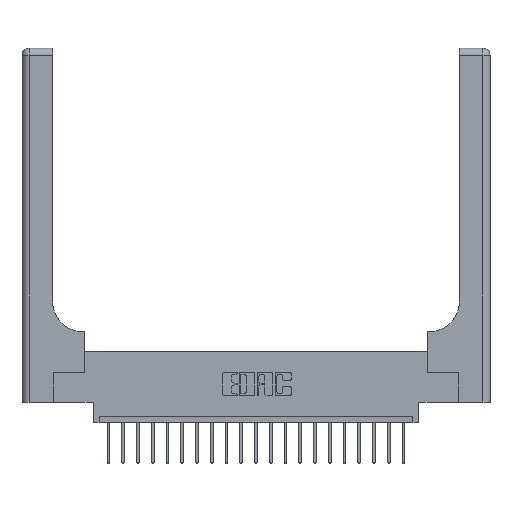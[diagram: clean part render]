
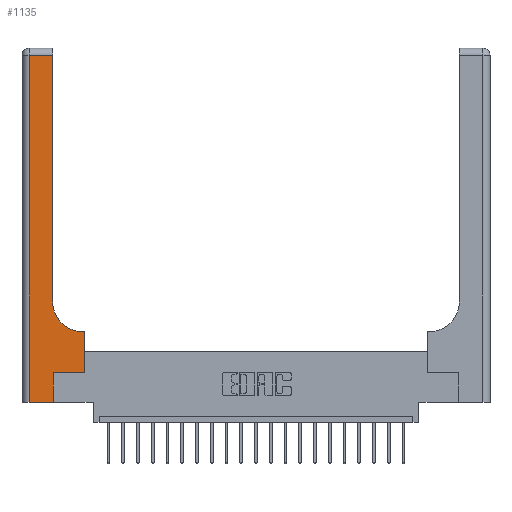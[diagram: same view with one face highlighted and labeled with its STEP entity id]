
A CAD part, top view. The second image highlights one B-rep face of the part: STEP entity #1135.
In plain terms, the highlighted planar face has unit normal (0, 0, 1).
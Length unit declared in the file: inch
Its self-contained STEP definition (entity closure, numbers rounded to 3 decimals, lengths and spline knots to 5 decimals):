
#511 = FACE_OUTER_BOUND ( 'NONE', #14439, .T. ) ;
#1135 = ADVANCED_FACE ( 'NONE', ( #511 ), #15843, .F. ) ;
#1681 = LINE ( 'NONE', #21353, #6158 ) ;
#1889 = CIRCLE ( 'NONE', #6447, 0.25 ) ;
#1968 = VECTOR ( 'NONE', #11763, 39.37008 ) ;
#2042 = CARTESIAN_POINT ( 'NONE',  ( 0.265, 0., 0.37 ) ) ;
#2161 = EDGE_CURVE ( 'NONE', #17078, #8652, #13279, .T. ) ;
#2388 = LINE ( 'NONE', #4135, #10143 ) ;
#3120 = ORIENTED_EDGE ( 'NONE', *, *, #17244, .T. ) ;
#3235 = VERTEX_POINT ( 'NONE', #18575 ) ;
#3741 = LINE ( 'NONE', #19071, #19484 ) ;
#4117 = CARTESIAN_POINT ( 'NONE',  ( 0.26, 2.94, 0.37 ) ) ;
#4135 = CARTESIAN_POINT ( 'NONE',  ( 0.265, 0.25, 0.37 ) ) ;
#4670 = VECTOR ( 'NONE', #9063, 39.37008 ) ;
#5354 = VERTEX_POINT ( 'NONE', #17963 ) ;
#5547 = EDGE_CURVE ( 'NONE', #6151, #3235, #2388, .T. ) ;
#5849 = VERTEX_POINT ( 'NONE', #21600 ) ;
#6035 = CARTESIAN_POINT ( 'NONE',  ( 0.26, 0.85, 0.37 ) ) ;
#6151 = VERTEX_POINT ( 'NONE', #16131 ) ;
#6158 = VECTOR ( 'NONE', #18116, 39.37008 ) ;
#6335 = AXIS2_PLACEMENT_3D ( 'NONE', #19245, #17715, #14543 ) ;
#6447 = AXIS2_PLACEMENT_3D ( 'NONE', #14978, #6541, #6746 ) ;
#6541 = DIRECTION ( 'NONE',  ( 0., 0., -1. ) ) ;
#6746 = DIRECTION ( 'NONE',  ( 1., 0., 0. ) ) ;
#8096 = EDGE_CURVE ( 'NONE', #8652, #5354, #3741, .T. ) ;
#8153 = ORIENTED_EDGE ( 'NONE', *, *, #15466, .T. ) ;
#8238 = CARTESIAN_POINT ( 'NONE',  ( 0., 2.94, 0.37 ) ) ;
#8451 = CARTESIAN_POINT ( 'NONE',  ( 0.265, 0., 0.37 ) ) ;
#8599 = VECTOR ( 'NONE', #13018, 39.37008 ) ;
#8652 = VERTEX_POINT ( 'NONE', #20749 ) ;
#8742 = LINE ( 'NONE', #17387, #4670 ) ;
#9063 = DIRECTION ( 'NONE',  ( 0., 1., 0. ) ) ;
#10143 = VECTOR ( 'NONE', #20635, 39.37008 ) ;
#10161 = EDGE_CURVE ( 'NONE', #17008, #6151, #20239, .T. ) ;
#10451 = DIRECTION ( 'NONE',  ( 0., 1., 0. ) ) ;
#11394 = CARTESIAN_POINT ( 'NONE',  ( 0.26, 0.6, 0.37 ) ) ;
#11500 = VERTEX_POINT ( 'NONE', #6035 ) ;
#11763 = DIRECTION ( 'NONE',  ( 0., 1., 0. ) ) ;
#13018 = DIRECTION ( 'NONE',  ( -1., 0., 0. ) ) ;
#13279 = LINE ( 'NONE', #8238, #16846 ) ;
#13583 = ORIENTED_EDGE ( 'NONE', *, *, #8096, .T. ) ;
#14439 = EDGE_LOOP ( 'NONE', ( #15401, #19778, #13583, #3120, #19257, #15819, #18914, #16451, #8153 ) ) ;
#14543 = DIRECTION ( 'NONE',  ( -1., 0., 0. ) ) ;
#14787 = CARTESIAN_POINT ( 'NONE',  ( 0.51, 0.6, 0.37 ) ) ;
#14978 = CARTESIAN_POINT ( 'NONE',  ( 0.51, 0.85, 0.37 ) ) ;
#15192 = EDGE_CURVE ( 'NONE', #3235, #5849, #8742, .T. ) ;
#15267 = LINE ( 'NONE', #11394, #8599 ) ;
#15401 = ORIENTED_EDGE ( 'NONE', *, *, #21593, .T. ) ;
#15462 = DIRECTION ( 'NONE',  ( 0., -1., 0. ) ) ;
#15466 = EDGE_CURVE ( 'NONE', #19342, #11500, #1889, .T. ) ;
#15819 = ORIENTED_EDGE ( 'NONE', *, *, #5547, .T. ) ;
#15843 = PLANE ( 'NONE',  #6335 ) ;
#16131 = CARTESIAN_POINT ( 'NONE',  ( 0.265, 0.25, 0.37 ) ) ;
#16451 = ORIENTED_EDGE ( 'NONE', *, *, #21181, .T. ) ;
#16846 = VECTOR ( 'NONE', #19437, 39.37008 ) ;
#17008 = VERTEX_POINT ( 'NONE', #2042 ) ;
#17078 = VERTEX_POINT ( 'NONE', #4117 ) ;
#17244 = EDGE_CURVE ( 'NONE', #5354, #17008, #1681, .T. ) ;
#17387 = CARTESIAN_POINT ( 'NONE',  ( 0.528, 0.25, 0.37 ) ) ;
#17715 = DIRECTION ( 'NONE',  ( 0., 0., -1. ) ) ;
#17963 = CARTESIAN_POINT ( 'NONE',  ( 0.06, 0., 0.37 ) ) ;
#18116 = DIRECTION ( 'NONE',  ( 1., 0., 0. ) ) ;
#18307 = LINE ( 'NONE', #20126, #1968 ) ;
#18575 = CARTESIAN_POINT ( 'NONE',  ( 0.528, 0.25, 0.37 ) ) ;
#18881 = VECTOR ( 'NONE', #10451, 39.37008 ) ;
#18914 = ORIENTED_EDGE ( 'NONE', *, *, #15192, .T. ) ;
#19071 = CARTESIAN_POINT ( 'NONE',  ( 0.06, 3., 0.37 ) ) ;
#19245 = CARTESIAN_POINT ( 'NONE',  ( 0., 3., 0.37 ) ) ;
#19257 = ORIENTED_EDGE ( 'NONE', *, *, #10161, .T. ) ;
#19342 = VERTEX_POINT ( 'NONE', #14787 ) ;
#19437 = DIRECTION ( 'NONE',  ( -1., 0., 0. ) ) ;
#19484 = VECTOR ( 'NONE', #15462, 39.37008 ) ;
#19778 = ORIENTED_EDGE ( 'NONE', *, *, #2161, .T. ) ;
#20126 = CARTESIAN_POINT ( 'NONE',  ( 0.26, 3., 0.37 ) ) ;
#20239 = LINE ( 'NONE', #8451, #18881 ) ;
#20635 = DIRECTION ( 'NONE',  ( 1., 0., 0. ) ) ;
#20749 = CARTESIAN_POINT ( 'NONE',  ( 0.06, 2.94, 0.37 ) ) ;
#21181 = EDGE_CURVE ( 'NONE', #5849, #19342, #15267, .T. ) ;
#21353 = CARTESIAN_POINT ( 'NONE',  ( 0., 0., 0.37 ) ) ;
#21593 = EDGE_CURVE ( 'NONE', #11500, #17078, #18307, .T. ) ;
#21600 = CARTESIAN_POINT ( 'NONE',  ( 0.528, 0.6, 0.37 ) ) ;
